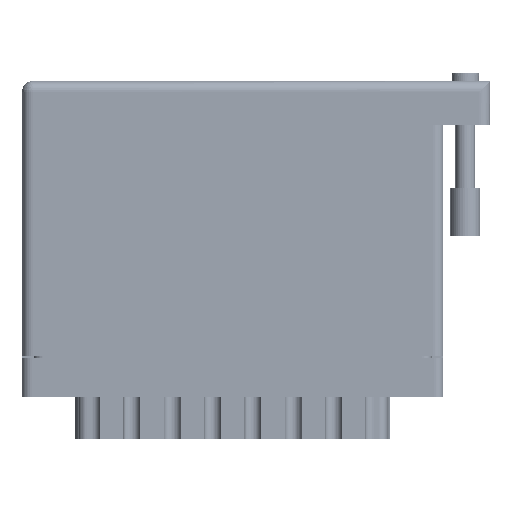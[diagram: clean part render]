
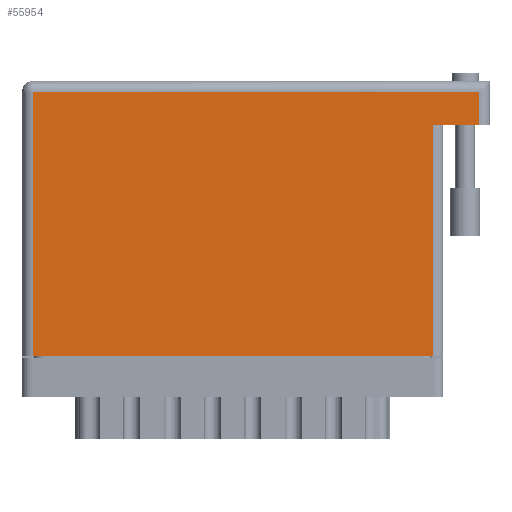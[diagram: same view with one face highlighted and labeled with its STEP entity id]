
A CAD part, front view. The second image highlights one B-rep face of the part: STEP entity #55954.
In plain terms, the highlighted face is planar.
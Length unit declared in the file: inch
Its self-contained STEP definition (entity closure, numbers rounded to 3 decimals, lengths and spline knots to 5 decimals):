
#122 = DIRECTION ( 'NONE',  ( -1., 0., 0. ) ) ;
#593 = CARTESIAN_POINT ( 'NONE',  ( 3.018, 1.495, 0. ) ) ;
#2817 = LINE ( 'NONE', #11306, #23902 ) ;
#2845 = ORIENTED_EDGE ( 'NONE', *, *, #9055, .T. ) ;
#2869 = LINE ( 'NONE', #55001, #6370 ) ;
#4293 = ORIENTED_EDGE ( 'NONE', *, *, #43837, .T. ) ;
#5448 = CARTESIAN_POINT ( 'NONE',  ( 2.648, 1.495, 0. ) ) ;
#5907 = ORIENTED_EDGE ( 'NONE', *, *, #66726, .T. ) ;
#6370 = VECTOR ( 'NONE', #15346, 39.37008 ) ;
#7611 = DIRECTION ( 'NONE',  ( -1., 0., 0. ) ) ;
#9055 = EDGE_CURVE ( 'NONE', #53508, #46961, #58667, .T. ) ;
#9408 = LINE ( 'NONE', #593, #63767 ) ;
#9877 = CARTESIAN_POINT ( 'NONE',  ( 2.648, 0., 0. ) ) ;
#11306 = CARTESIAN_POINT ( 'NONE',  ( 2.648, 1.495, 0. ) ) ;
#11431 = CARTESIAN_POINT ( 'NONE',  ( 0.07, 0., 0. ) ) ;
#11858 = CARTESIAN_POINT ( 'NONE',  ( 2.948, 1.705, 0. ) ) ;
#12487 = VECTOR ( 'NONE', #22579, 39.37008 ) ;
#15346 = DIRECTION ( 'NONE',  ( 1., 0., 0. ) ) ;
#17482 = DIRECTION ( 'NONE',  ( 0., 1., 0. ) ) ;
#20186 = VERTEX_POINT ( 'NONE', #9877 ) ;
#20528 = DIRECTION ( 'NONE',  ( 0., -1., 0. ) ) ;
#20678 = VERTEX_POINT ( 'NONE', #5448 ) ;
#21608 = CARTESIAN_POINT ( 'NONE',  ( 0., 1.705, 0. ) ) ;
#22579 = DIRECTION ( 'NONE',  ( -1., 0., 0. ) ) ;
#22868 = CARTESIAN_POINT ( 'NONE',  ( 0.07, 1.705, 0. ) ) ;
#23622 = CARTESIAN_POINT ( 'NONE',  ( 2.948, 1.775, 0. ) ) ;
#23902 = VECTOR ( 'NONE', #56841, 39.37008 ) ;
#24485 = VECTOR ( 'NONE', #20528, 39.37008 ) ;
#25034 = EDGE_CURVE ( 'NONE', #59904, #20678, #9408, .T. ) ;
#25086 = PLANE ( 'NONE',  #65274 ) ;
#27418 = LINE ( 'NONE', #21608, #12487 ) ;
#30165 = VECTOR ( 'NONE', #17482, 39.37008 ) ;
#41517 = DIRECTION ( 'NONE',  ( 0., 0., -1. ) ) ;
#42852 = VERTEX_POINT ( 'NONE', #11858 ) ;
#43837 = EDGE_CURVE ( 'NONE', #42852, #53508, #27418, .T. ) ;
#46350 = EDGE_LOOP ( 'NONE', ( #5907, #57550, #53251, #52667, #4293, #2845 ) ) ;
#46961 = VERTEX_POINT ( 'NONE', #11431 ) ;
#47591 = CARTESIAN_POINT ( 'NONE',  ( 0., 1.775, 0. ) ) ;
#48466 = CARTESIAN_POINT ( 'NONE',  ( 0.07, 0., 0. ) ) ;
#52667 = ORIENTED_EDGE ( 'NONE', *, *, #62757, .T. ) ;
#53251 = ORIENTED_EDGE ( 'NONE', *, *, #25034, .F. ) ;
#53508 = VERTEX_POINT ( 'NONE', #22868 ) ;
#55001 = CARTESIAN_POINT ( 'NONE',  ( 0., 0., 0. ) ) ;
#55954 = ADVANCED_FACE ( 'NONE', ( #69388 ), #25086, .F. ) ;
#56841 = DIRECTION ( 'NONE',  ( 0., 1., 0. ) ) ;
#57550 = ORIENTED_EDGE ( 'NONE', *, *, #67577, .T. ) ;
#58180 = LINE ( 'NONE', #23622, #30165 ) ;
#58667 = LINE ( 'NONE', #48466, #24485 ) ;
#59523 = CARTESIAN_POINT ( 'NONE',  ( 2.948, 1.495, 0. ) ) ;
#59904 = VERTEX_POINT ( 'NONE', #59523 ) ;
#62757 = EDGE_CURVE ( 'NONE', #59904, #42852, #58180, .T. ) ;
#63767 = VECTOR ( 'NONE', #122, 39.37008 ) ;
#65274 = AXIS2_PLACEMENT_3D ( 'NONE', #47591, #41517, #7611 ) ;
#66726 = EDGE_CURVE ( 'NONE', #46961, #20186, #2869, .T. ) ;
#67577 = EDGE_CURVE ( 'NONE', #20186, #20678, #2817, .T. ) ;
#69388 = FACE_OUTER_BOUND ( 'NONE', #46350, .T. ) ;
